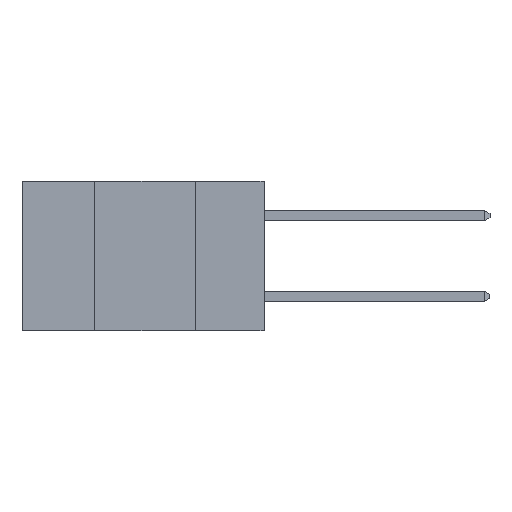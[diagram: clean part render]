
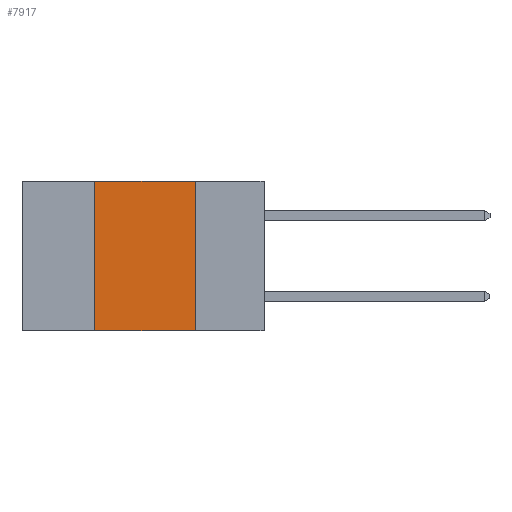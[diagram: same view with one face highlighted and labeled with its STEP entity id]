
A CAD part, left-side view. The second image highlights one B-rep face of the part: STEP entity #7917.
In plain terms, the highlighted planar face has unit normal (-1, 0, 0).
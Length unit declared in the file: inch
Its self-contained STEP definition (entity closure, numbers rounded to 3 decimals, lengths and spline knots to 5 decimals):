
#215 = EDGE_LOOP ( 'NONE', ( #11401, #13404, #5083, #5414 ) ) ;
#2669 = CARTESIAN_POINT ( 'NONE',  ( 0., 0.17, 0. ) ) ;
#5083 = ORIENTED_EDGE ( 'NONE', *, *, #12736, .F. ) ;
#5166 = VECTOR ( 'NONE', #9240, 39.37008 ) ;
#5414 = ORIENTED_EDGE ( 'NONE', *, *, #9693, .T. ) ;
#6122 = CARTESIAN_POINT ( 'NONE',  ( 0., 0.42, 0. ) ) ;
#6691 = VERTEX_POINT ( 'NONE', #9017 ) ;
#7917 = ADVANCED_FACE ( 'NONE', ( #9699 ), #13129, .F. ) ;
#7956 = CARTESIAN_POINT ( 'NONE',  ( 0., 0.6, -0.37 ) ) ;
#8146 = LINE ( 'NONE', #12592, #11281 ) ;
#8478 = VECTOR ( 'NONE', #15479, 39.37008 ) ;
#9017 = CARTESIAN_POINT ( 'NONE',  ( 0., 0.42, 0. ) ) ;
#9240 = DIRECTION ( 'NONE',  ( 0., -1., 0. ) ) ;
#9693 = EDGE_CURVE ( 'NONE', #11834, #11678, #15390, .T. ) ;
#9699 = FACE_OUTER_BOUND ( 'NONE', #215, .T. ) ;
#10309 = LINE ( 'NONE', #6122, #12977 ) ;
#10327 = DIRECTION ( 'NONE',  ( 0., 0., 1. ) ) ;
#10942 = CARTESIAN_POINT ( 'NONE',  ( 0., 0.17, -0.37 ) ) ;
#11281 = VECTOR ( 'NONE', #16298, 39.37008 ) ;
#11401 = ORIENTED_EDGE ( 'NONE', *, *, #16344, .F. ) ;
#11587 = CARTESIAN_POINT ( 'NONE',  ( 0., 0.17, 0. ) ) ;
#11678 = VERTEX_POINT ( 'NONE', #10942 ) ;
#11834 = VERTEX_POINT ( 'NONE', #12548 ) ;
#12548 = CARTESIAN_POINT ( 'NONE',  ( 0., 0.42, -0.37 ) ) ;
#12592 = CARTESIAN_POINT ( 'NONE',  ( 0., 0.6, 0. ) ) ;
#12736 = EDGE_CURVE ( 'NONE', #11834, #6691, #10309, .T. ) ;
#12977 = VECTOR ( 'NONE', #10327, 39.37008 ) ;
#13062 = DIRECTION ( 'NONE',  ( 0., 0., -1. ) ) ;
#13083 = DIRECTION ( 'NONE',  ( 1., 0., 0. ) ) ;
#13114 = CARTESIAN_POINT ( 'NONE',  ( 0., 0.6, 0. ) ) ;
#13129 = PLANE ( 'NONE',  #15161 ) ;
#13365 = VERTEX_POINT ( 'NONE', #11587 ) ;
#13404 = ORIENTED_EDGE ( 'NONE', *, *, #14346, .F. ) ;
#14346 = EDGE_CURVE ( 'NONE', #6691, #13365, #8146, .T. ) ;
#15161 = AXIS2_PLACEMENT_3D ( 'NONE', #13114, #13083, #13062 ) ;
#15364 = LINE ( 'NONE', #2669, #8478 ) ;
#15390 = LINE ( 'NONE', #7956, #5166 ) ;
#15479 = DIRECTION ( 'NONE',  ( 0., 0., -1. ) ) ;
#16298 = DIRECTION ( 'NONE',  ( 0., -1., 0. ) ) ;
#16344 = EDGE_CURVE ( 'NONE', #13365, #11678, #15364, .T. ) ;
